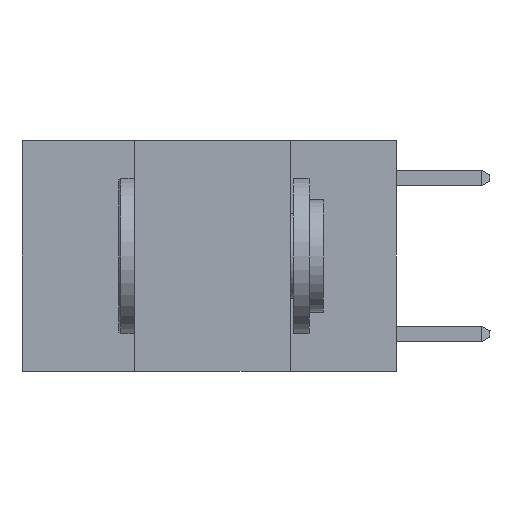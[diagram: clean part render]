
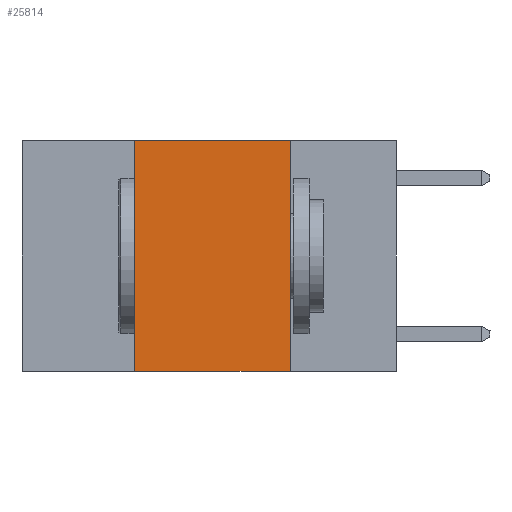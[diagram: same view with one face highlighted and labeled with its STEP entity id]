
A CAD part, left-side view. The second image highlights one B-rep face of the part: STEP entity #25814.
In plain terms, the highlighted planar face has unit normal (-1, 0, 0).
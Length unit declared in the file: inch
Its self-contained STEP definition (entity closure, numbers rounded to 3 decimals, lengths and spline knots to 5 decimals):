
#765 = VECTOR ( 'NONE', #17152, 39.37008 ) ;
#2221 = DIRECTION ( 'NONE',  ( 1., 0., 0. ) ) ;
#3221 = ORIENTED_EDGE ( 'NONE', *, *, #31895, .T. ) ;
#4630 = EDGE_CURVE ( 'NONE', #14397, #14386, #7523, .T. ) ;
#4727 = PLANE ( 'NONE',  #16799 ) ;
#4875 = CARTESIAN_POINT ( 'NONE',  ( 0., 0.6, 0. ) ) ;
#7211 = CARTESIAN_POINT ( 'NONE',  ( 0., 0.6, 0. ) ) ;
#7523 = LINE ( 'NONE', #4875, #765 ) ;
#7643 = VERTEX_POINT ( 'NONE', #20872 ) ;
#7843 = EDGE_CURVE ( 'NONE', #14386, #7643, #24511, .T. ) ;
#8075 = VERTEX_POINT ( 'NONE', #32474 ) ;
#8783 = DIRECTION ( 'NONE',  ( 0., -1., 0. ) ) ;
#8894 = DIRECTION ( 'NONE',  ( 0., 0., -1. ) ) ;
#11103 = VECTOR ( 'NONE', #20175, 39.37008 ) ;
#12042 = CARTESIAN_POINT ( 'NONE',  ( 0., 0.17, 0. ) ) ;
#12370 = CARTESIAN_POINT ( 'NONE',  ( 0., 0.42, 0. ) ) ;
#13998 = ORIENTED_EDGE ( 'NONE', *, *, #4630, .F. ) ;
#14386 = VERTEX_POINT ( 'NONE', #32632 ) ;
#14397 = VERTEX_POINT ( 'NONE', #12370 ) ;
#14422 = LINE ( 'NONE', #21403, #29314 ) ;
#15498 = ORIENTED_EDGE ( 'NONE', *, *, #7843, .F. ) ;
#15522 = EDGE_LOOP ( 'NONE', ( #15498, #13998, #17824, #3221 ) ) ;
#16799 = AXIS2_PLACEMENT_3D ( 'NONE', #7211, #2221, #27980 ) ;
#17152 = DIRECTION ( 'NONE',  ( 0., -1., 0. ) ) ;
#17654 = FACE_OUTER_BOUND ( 'NONE', #15522, .T. ) ;
#17824 = ORIENTED_EDGE ( 'NONE', *, *, #18260, .F. ) ;
#18087 = VECTOR ( 'NONE', #8894, 39.37008 ) ;
#18260 = EDGE_CURVE ( 'NONE', #8075, #14397, #22681, .T. ) ;
#20175 = DIRECTION ( 'NONE',  ( 0., 0., 1. ) ) ;
#20872 = CARTESIAN_POINT ( 'NONE',  ( 0., 0.17, -0.37 ) ) ;
#21403 = CARTESIAN_POINT ( 'NONE',  ( 0., 0.6, -0.37 ) ) ;
#22681 = LINE ( 'NONE', #26799, #11103 ) ;
#24511 = LINE ( 'NONE', #12042, #18087 ) ;
#25814 = ADVANCED_FACE ( 'NONE', ( #17654 ), #4727, .F. ) ;
#26799 = CARTESIAN_POINT ( 'NONE',  ( 0., 0.42, 0. ) ) ;
#27980 = DIRECTION ( 'NONE',  ( 0., 0., -1. ) ) ;
#29314 = VECTOR ( 'NONE', #8783, 39.37008 ) ;
#31895 = EDGE_CURVE ( 'NONE', #8075, #7643, #14422, .T. ) ;
#32474 = CARTESIAN_POINT ( 'NONE',  ( 0., 0.42, -0.37 ) ) ;
#32632 = CARTESIAN_POINT ( 'NONE',  ( 0., 0.17, 0. ) ) ;
